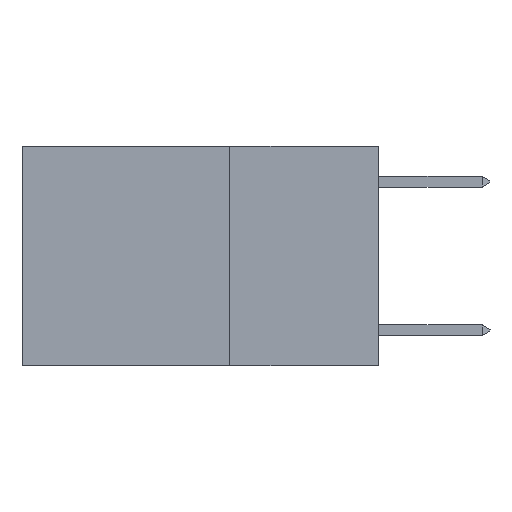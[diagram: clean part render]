
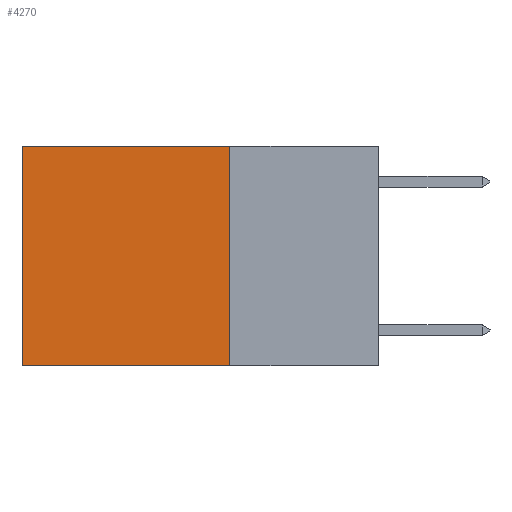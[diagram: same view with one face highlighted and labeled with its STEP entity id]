
A CAD part, left-side view. The second image highlights one B-rep face of the part: STEP entity #4270.
In plain terms, the highlighted planar face has unit normal (-1, 0, 0).
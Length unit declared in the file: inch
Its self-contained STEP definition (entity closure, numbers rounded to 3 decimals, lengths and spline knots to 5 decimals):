
#225 = DIRECTION ( 'NONE',  ( 0., 0., -1. ) ) ;
#1424 = CARTESIAN_POINT ( 'NONE',  ( 0.2625, 0.6, 0. ) ) ;
#1566 = CARTESIAN_POINT ( 'NONE',  ( 0.2625, 0.25, 0. ) ) ;
#1887 = CARTESIAN_POINT ( 'NONE',  ( 0.2625, 0.6, -0.37 ) ) ;
#3100 = ORIENTED_EDGE ( 'NONE', *, *, #16626, .F. ) ;
#4270 = ADVANCED_FACE ( 'NONE', ( #11775 ), #6131, .F. ) ;
#5730 = EDGE_LOOP ( 'NONE', ( #23226, #21059, #3100, #11885 ) ) ;
#6131 = PLANE ( 'NONE',  #18132 ) ;
#8363 = DIRECTION ( 'NONE',  ( 0., 0., -1. ) ) ;
#8597 = VERTEX_POINT ( 'NONE', #14284 ) ;
#10672 = VECTOR ( 'NONE', #28123, 39.37008 ) ;
#11775 = FACE_OUTER_BOUND ( 'NONE', #5730, .T. ) ;
#11885 = ORIENTED_EDGE ( 'NONE', *, *, #21748, .T. ) ;
#12685 = VERTEX_POINT ( 'NONE', #1424 ) ;
#12863 = DIRECTION ( 'NONE',  ( 0., 0., -1. ) ) ;
#14273 = LINE ( 'NONE', #26589, #19468 ) ;
#14284 = CARTESIAN_POINT ( 'NONE',  ( 0.2625, 0.25, -0.37 ) ) ;
#14884 = LINE ( 'NONE', #23899, #20068 ) ;
#16626 = EDGE_CURVE ( 'NONE', #28257, #8597, #23988, .T. ) ;
#17417 = VECTOR ( 'NONE', #225, 39.37008 ) ;
#18116 = CARTESIAN_POINT ( 'NONE',  ( 0.2625, 0.25, 0. ) ) ;
#18132 = AXIS2_PLACEMENT_3D ( 'NONE', #1566, #21612, #8363 ) ;
#18467 = VERTEX_POINT ( 'NONE', #1887 ) ;
#18584 = EDGE_CURVE ( 'NONE', #8597, #18467, #14273, .T. ) ;
#19468 = VECTOR ( 'NONE', #22291, 39.37008 ) ;
#20068 = VECTOR ( 'NONE', #12863, 39.37008 ) ;
#21059 = ORIENTED_EDGE ( 'NONE', *, *, #18584, .F. ) ;
#21119 = EDGE_CURVE ( 'NONE', #12685, #18467, #14884, .T. ) ;
#21343 = CARTESIAN_POINT ( 'NONE',  ( 0.2625, 0.25, 0. ) ) ;
#21612 = DIRECTION ( 'NONE',  ( 1., 0., 0. ) ) ;
#21748 = EDGE_CURVE ( 'NONE', #28257, #12685, #28232, .T. ) ;
#22291 = DIRECTION ( 'NONE',  ( 0., 1., 0. ) ) ;
#23226 = ORIENTED_EDGE ( 'NONE', *, *, #21119, .T. ) ;
#23899 = CARTESIAN_POINT ( 'NONE',  ( 0.2625, 0.6, 0. ) ) ;
#23988 = LINE ( 'NONE', #18116, #17417 ) ;
#25960 = CARTESIAN_POINT ( 'NONE',  ( 0.2625, 0.25, 0. ) ) ;
#26589 = CARTESIAN_POINT ( 'NONE',  ( 0.2625, 0.25, -0.37 ) ) ;
#28123 = DIRECTION ( 'NONE',  ( 0., 1., 0. ) ) ;
#28232 = LINE ( 'NONE', #25960, #10672 ) ;
#28257 = VERTEX_POINT ( 'NONE', #21343 ) ;
